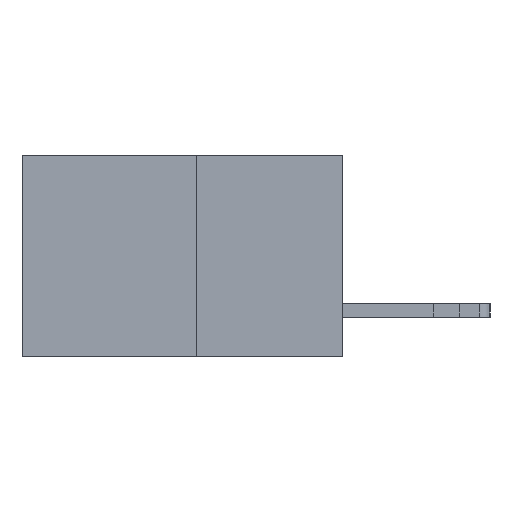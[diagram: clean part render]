
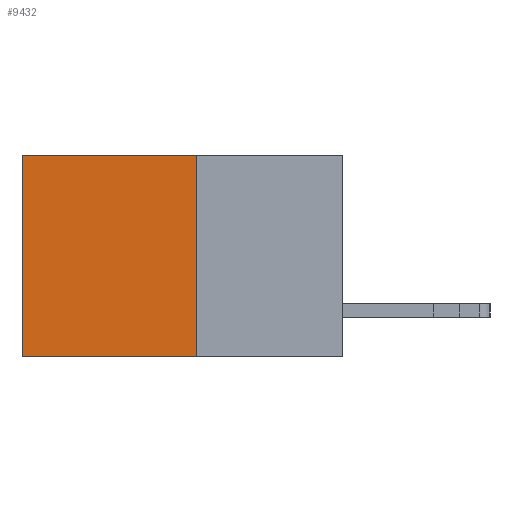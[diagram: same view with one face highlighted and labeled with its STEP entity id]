
A CAD part, left-side view. The second image highlights one B-rep face of the part: STEP entity #9432.
In plain terms, the highlighted planar face has unit normal (-1, 0, 0).
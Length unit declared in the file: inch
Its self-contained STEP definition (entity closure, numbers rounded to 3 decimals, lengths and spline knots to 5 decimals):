
#221 = CARTESIAN_POINT ( 'NONE',  ( 0.277, 0.59, 0. ) ) ;
#1849 = VERTEX_POINT ( 'NONE', #4498 ) ;
#2027 = ORIENTED_EDGE ( 'NONE', *, *, #10093, .F. ) ;
#3363 = ORIENTED_EDGE ( 'NONE', *, *, #3629, .T. ) ;
#3629 = EDGE_CURVE ( 'NONE', #14919, #9943, #13998, .T. ) ;
#3890 = EDGE_CURVE ( 'NONE', #9943, #1849, #4349, .T. ) ;
#4349 = LINE ( 'NONE', #11443, #10965 ) ;
#4498 = CARTESIAN_POINT ( 'NONE',  ( 0.277, 0.59, -0.37 ) ) ;
#4823 = DIRECTION ( 'NONE',  ( 0., 0., -1. ) ) ;
#4842 = DIRECTION ( 'NONE',  ( 1., 0., 0. ) ) ;
#4862 = CARTESIAN_POINT ( 'NONE',  ( 0.277, 0.27, -0.37 ) ) ;
#4882 = PLANE ( 'NONE',  #12002 ) ;
#5944 = CARTESIAN_POINT ( 'NONE',  ( 0.277, 0.27, -0.37 ) ) ;
#7246 = DIRECTION ( 'NONE',  ( 0., 1., 0. ) ) ;
#7954 = FACE_OUTER_BOUND ( 'NONE', #15873, .T. ) ;
#8490 = VECTOR ( 'NONE', #15340, 39.37008 ) ;
#9432 = ADVANCED_FACE ( 'NONE', ( #7954 ), #4882, .F. ) ;
#9943 = VERTEX_POINT ( 'NONE', #221 ) ;
#10093 = EDGE_CURVE ( 'NONE', #10717, #1849, #11494, .T. ) ;
#10645 = VECTOR ( 'NONE', #7246, 39.37008 ) ;
#10717 = VERTEX_POINT ( 'NONE', #17157 ) ;
#10965 = VECTOR ( 'NONE', #11400, 39.37008 ) ;
#10983 = VECTOR ( 'NONE', #14889, 39.37008 ) ;
#11400 = DIRECTION ( 'NONE',  ( 0., 0., -1. ) ) ;
#11443 = CARTESIAN_POINT ( 'NONE',  ( 0.277, 0.59, -0.37 ) ) ;
#11494 = LINE ( 'NONE', #5944, #10645 ) ;
#11539 = CARTESIAN_POINT ( 'NONE',  ( 0.277, 0.27, -0.37 ) ) ;
#12002 = AXIS2_PLACEMENT_3D ( 'NONE', #4862, #4842, #4823 ) ;
#12044 = LINE ( 'NONE', #11539, #8490 ) ;
#12073 = EDGE_CURVE ( 'NONE', #14919, #10717, #12044, .T. ) ;
#12958 = ORIENTED_EDGE ( 'NONE', *, *, #3890, .T. ) ;
#13998 = LINE ( 'NONE', #14926, #10983 ) ;
#14508 = ORIENTED_EDGE ( 'NONE', *, *, #12073, .F. ) ;
#14889 = DIRECTION ( 'NONE',  ( 0., 1., 0. ) ) ;
#14919 = VERTEX_POINT ( 'NONE', #16462 ) ;
#14926 = CARTESIAN_POINT ( 'NONE',  ( 0.277, 0.27, 0. ) ) ;
#15340 = DIRECTION ( 'NONE',  ( 0., 0., -1. ) ) ;
#15873 = EDGE_LOOP ( 'NONE', ( #12958, #2027, #14508, #3363 ) ) ;
#16462 = CARTESIAN_POINT ( 'NONE',  ( 0.277, 0.27, 0. ) ) ;
#17157 = CARTESIAN_POINT ( 'NONE',  ( 0.277, 0.27, -0.37 ) ) ;
